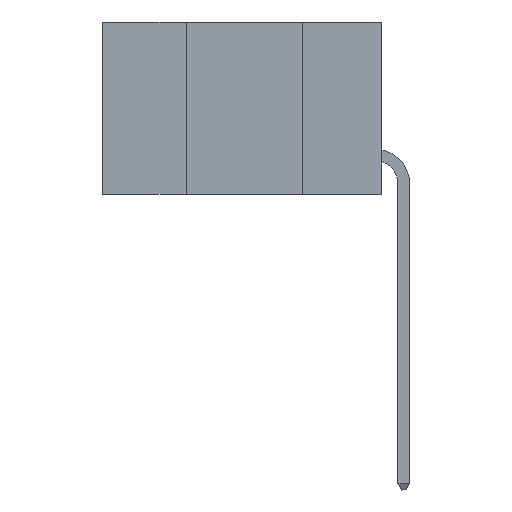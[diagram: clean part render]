
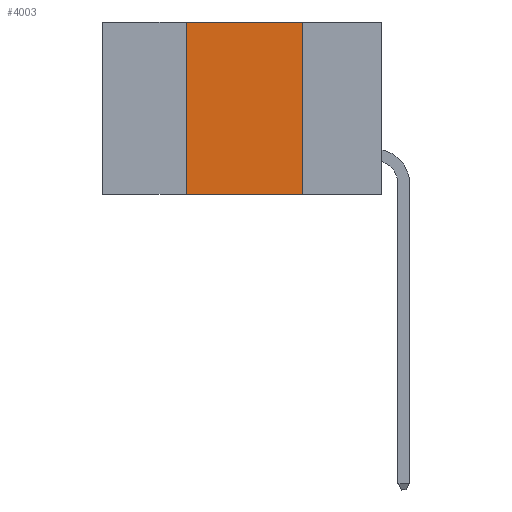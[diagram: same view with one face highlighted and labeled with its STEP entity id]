
A CAD part, left-side view. The second image highlights one B-rep face of the part: STEP entity #4003.
In plain terms, the highlighted planar face has unit normal (-1, 0, 0).
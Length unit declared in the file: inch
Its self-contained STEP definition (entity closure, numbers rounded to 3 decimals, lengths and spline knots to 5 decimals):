
#402 = EDGE_LOOP ( 'NONE', ( #13315, #6816, #11768, #13884 ) ) ;
#528 = VERTEX_POINT ( 'NONE', #633 ) ;
#633 = CARTESIAN_POINT ( 'NONE',  ( 0., 0.42, -0.37 ) ) ;
#789 = CARTESIAN_POINT ( 'NONE',  ( 0., 0.6, -0.37 ) ) ;
#1460 = LINE ( 'NONE', #789, #2754 ) ;
#2108 = DIRECTION ( 'NONE',  ( 0., 0., -1. ) ) ;
#2205 = LINE ( 'NONE', #9872, #11568 ) ;
#2754 = VECTOR ( 'NONE', #10558, 39.37008 ) ;
#4003 = ADVANCED_FACE ( 'NONE', ( #7953 ), #11826, .F. ) ;
#5841 = CARTESIAN_POINT ( 'NONE',  ( 0., 0.6, 0. ) ) ;
#6119 = DIRECTION ( 'NONE',  ( 0., -1., 0. ) ) ;
#6183 = DIRECTION ( 'NONE',  ( 0., 0., -1. ) ) ;
#6228 = CARTESIAN_POINT ( 'NONE',  ( 0., 0.17, 0. ) ) ;
#6713 = CARTESIAN_POINT ( 'NONE',  ( 0., 0.42, 0. ) ) ;
#6816 = ORIENTED_EDGE ( 'NONE', *, *, #8697, .F. ) ;
#7332 = DIRECTION ( 'NONE',  ( 1., 0., 0. ) ) ;
#7953 = FACE_OUTER_BOUND ( 'NONE', #402, .T. ) ;
#8067 = VERTEX_POINT ( 'NONE', #6228 ) ;
#8091 = LINE ( 'NONE', #12322, #15502 ) ;
#8224 = CARTESIAN_POINT ( 'NONE',  ( 0., 0.6, 0. ) ) ;
#8632 = VERTEX_POINT ( 'NONE', #6713 ) ;
#8697 = EDGE_CURVE ( 'NONE', #8632, #8067, #11059, .T. ) ;
#9872 = CARTESIAN_POINT ( 'NONE',  ( 0., 0.17, 0. ) ) ;
#9965 = DIRECTION ( 'NONE',  ( 0., 0., 1. ) ) ;
#10083 = CARTESIAN_POINT ( 'NONE',  ( 0., 0.17, -0.37 ) ) ;
#10558 = DIRECTION ( 'NONE',  ( 0., -1., 0. ) ) ;
#11059 = LINE ( 'NONE', #5841, #13136 ) ;
#11568 = VECTOR ( 'NONE', #6183, 39.37008 ) ;
#11719 = EDGE_CURVE ( 'NONE', #528, #8632, #8091, .T. ) ;
#11768 = ORIENTED_EDGE ( 'NONE', *, *, #11719, .F. ) ;
#11826 = PLANE ( 'NONE',  #14698 ) ;
#12322 = CARTESIAN_POINT ( 'NONE',  ( 0., 0.42, 0. ) ) ;
#13136 = VECTOR ( 'NONE', #6119, 39.37008 ) ;
#13315 = ORIENTED_EDGE ( 'NONE', *, *, #14844, .F. ) ;
#13863 = VERTEX_POINT ( 'NONE', #10083 ) ;
#13884 = ORIENTED_EDGE ( 'NONE', *, *, #14704, .T. ) ;
#14698 = AXIS2_PLACEMENT_3D ( 'NONE', #8224, #7332, #2108 ) ;
#14704 = EDGE_CURVE ( 'NONE', #528, #13863, #1460, .T. ) ;
#14844 = EDGE_CURVE ( 'NONE', #8067, #13863, #2205, .T. ) ;
#15502 = VECTOR ( 'NONE', #9965, 39.37008 ) ;
